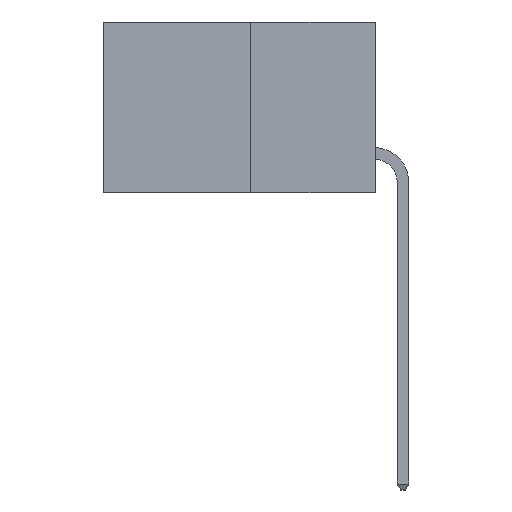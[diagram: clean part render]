
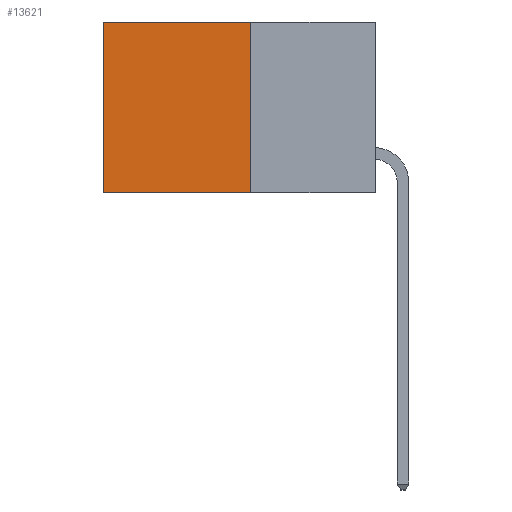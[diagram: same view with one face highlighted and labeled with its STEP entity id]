
A CAD part, left-side view. The second image highlights one B-rep face of the part: STEP entity #13621.
In plain terms, the highlighted planar face has unit normal (-1, 0, 0).
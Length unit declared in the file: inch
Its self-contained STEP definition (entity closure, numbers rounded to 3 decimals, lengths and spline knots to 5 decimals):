
#459 = ORIENTED_EDGE ( 'NONE', *, *, #15581, .F. ) ;
#942 = VECTOR ( 'NONE', #4114, 39.37008 ) ;
#1030 = ORIENTED_EDGE ( 'NONE', *, *, #4372, .T. ) ;
#1828 = CARTESIAN_POINT ( 'NONE',  ( 0.277, 0.27, -0.37 ) ) ;
#2540 = CARTESIAN_POINT ( 'NONE',  ( 0.277, 0.27, -0.37 ) ) ;
#3190 = CARTESIAN_POINT ( 'NONE',  ( 0.277, 0.27, 0. ) ) ;
#3335 = AXIS2_PLACEMENT_3D ( 'NONE', #2540, #7037, #22293 ) ;
#3358 = DIRECTION ( 'NONE',  ( 0., 1., 0. ) ) ;
#4114 = DIRECTION ( 'NONE',  ( 0., 0., -1. ) ) ;
#4372 = EDGE_CURVE ( 'NONE', #12322, #6431, #20952, .T. ) ;
#4799 = FACE_OUTER_BOUND ( 'NONE', #25796, .T. ) ;
#6431 = VERTEX_POINT ( 'NONE', #8411 ) ;
#7037 = DIRECTION ( 'NONE',  ( 1., 0., 0. ) ) ;
#7472 = EDGE_CURVE ( 'NONE', #6431, #14037, #11599, .T. ) ;
#7851 = ORIENTED_EDGE ( 'NONE', *, *, #22654, .F. ) ;
#8411 = CARTESIAN_POINT ( 'NONE',  ( 0.277, 0.59, 0. ) ) ;
#8505 = VECTOR ( 'NONE', #25911, 39.37008 ) ;
#9163 = VERTEX_POINT ( 'NONE', #26157 ) ;
#11599 = LINE ( 'NONE', #22945, #22539 ) ;
#12322 = VERTEX_POINT ( 'NONE', #19509 ) ;
#12831 = CARTESIAN_POINT ( 'NONE',  ( 0.277, 0.27, -0.37 ) ) ;
#13088 = ORIENTED_EDGE ( 'NONE', *, *, #7472, .T. ) ;
#13621 = ADVANCED_FACE ( 'NONE', ( #4799 ), #26441, .F. ) ;
#14037 = VERTEX_POINT ( 'NONE', #23410 ) ;
#14209 = DIRECTION ( 'NONE',  ( 0., 0., -1. ) ) ;
#14234 = LINE ( 'NONE', #12831, #8505 ) ;
#15105 = VECTOR ( 'NONE', #3358, 39.37008 ) ;
#15581 = EDGE_CURVE ( 'NONE', #12322, #9163, #17881, .T. ) ;
#17881 = LINE ( 'NONE', #1828, #942 ) ;
#19509 = CARTESIAN_POINT ( 'NONE',  ( 0.277, 0.27, 0. ) ) ;
#20952 = LINE ( 'NONE', #3190, #15105 ) ;
#22293 = DIRECTION ( 'NONE',  ( 0., 0., -1. ) ) ;
#22539 = VECTOR ( 'NONE', #14209, 39.37008 ) ;
#22654 = EDGE_CURVE ( 'NONE', #9163, #14037, #14234, .T. ) ;
#22945 = CARTESIAN_POINT ( 'NONE',  ( 0.277, 0.59, -0.37 ) ) ;
#23410 = CARTESIAN_POINT ( 'NONE',  ( 0.277, 0.59, -0.37 ) ) ;
#25796 = EDGE_LOOP ( 'NONE', ( #13088, #7851, #459, #1030 ) ) ;
#25911 = DIRECTION ( 'NONE',  ( 0., 1., 0. ) ) ;
#26157 = CARTESIAN_POINT ( 'NONE',  ( 0.277, 0.27, -0.37 ) ) ;
#26441 = PLANE ( 'NONE',  #3335 ) ;
